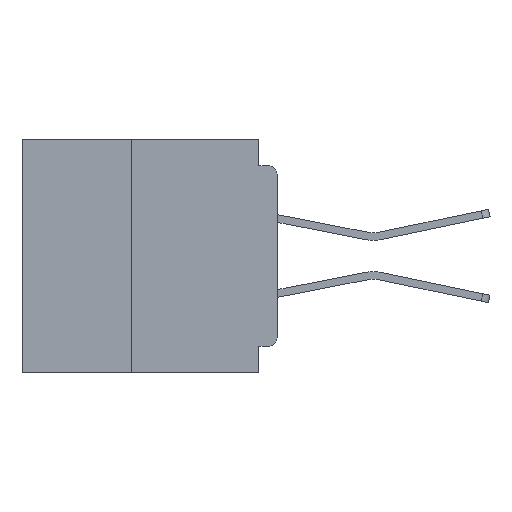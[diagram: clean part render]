
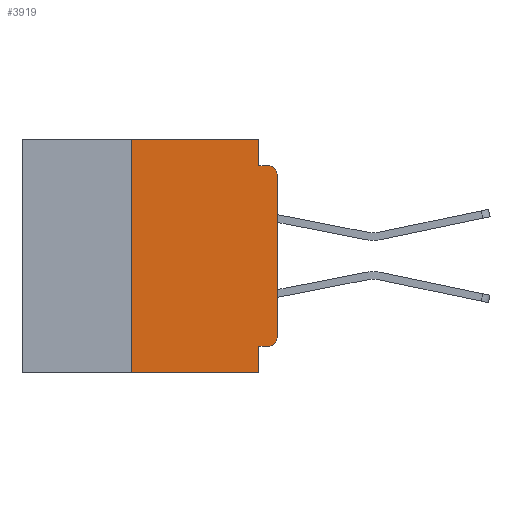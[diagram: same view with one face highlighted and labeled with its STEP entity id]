
A CAD part, left-side view. The second image highlights one B-rep face of the part: STEP entity #3919.
In plain terms, the highlighted planar face has unit normal (-1, 0, 0).
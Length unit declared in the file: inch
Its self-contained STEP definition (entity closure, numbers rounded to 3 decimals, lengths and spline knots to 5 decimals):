
#344 = DIRECTION ( 'NONE',  ( 0., 0., -1. ) ) ;
#1067 = CARTESIAN_POINT ( 'NONE',  ( 0., 0., -0.06 ) ) ;
#1111 = VECTOR ( 'NONE', #30399, 39.37008 ) ;
#1679 = VECTOR ( 'NONE', #43311, 39.37008 ) ;
#3634 = ORIENTED_EDGE ( 'NONE', *, *, #13479, .F. ) ;
#3635 = DIRECTION ( 'NONE',  ( 0., 0., 1. ) ) ;
#3919 = ADVANCED_FACE ( 'NONE', ( #28523 ), #49571, .F. ) ;
#3996 = VERTEX_POINT ( 'NONE', #1067 ) ;
#8938 = LINE ( 'NONE', #18709, #19869 ) ;
#9165 = ORIENTED_EDGE ( 'NONE', *, *, #11677, .T. ) ;
#9570 = VERTEX_POINT ( 'NONE', #10868 ) ;
#10157 = VERTEX_POINT ( 'NONE', #14753 ) ;
#10261 = VECTOR ( 'NONE', #28256, 39.37008 ) ;
#10330 = VERTEX_POINT ( 'NONE', #11657 ) ;
#10868 = CARTESIAN_POINT ( 'NONE',  ( 0., 0.031, -0.045 ) ) ;
#11498 = CARTESIAN_POINT ( 'NONE',  ( 0., 0.031, 0. ) ) ;
#11657 = CARTESIAN_POINT ( 'NONE',  ( 0., 0.25, -0.4 ) ) ;
#11677 = EDGE_CURVE ( 'NONE', #28107, #3996, #35769, .T. ) ;
#12485 = CARTESIAN_POINT ( 'NONE',  ( 0., 0., -0.355 ) ) ;
#13479 = EDGE_CURVE ( 'NONE', #10157, #34674, #44838, .T. ) ;
#14753 = CARTESIAN_POINT ( 'NONE',  ( 0., 0.031, -0.355 ) ) ;
#15132 = CIRCLE ( 'NONE', #24941, 0.015 ) ;
#15340 = VECTOR ( 'NONE', #19314, 39.37008 ) ;
#17883 = LINE ( 'NONE', #39965, #27533 ) ;
#17892 = CARTESIAN_POINT ( 'NONE',  ( 0., 0.031, -0.4 ) ) ;
#18213 = CARTESIAN_POINT ( 'NONE',  ( 0., 0.015, -0.06 ) ) ;
#18709 = CARTESIAN_POINT ( 'NONE',  ( 0., 0.437, -0.4 ) ) ;
#19314 = DIRECTION ( 'NONE',  ( 0., 0., -1. ) ) ;
#19401 = VERTEX_POINT ( 'NONE', #26778 ) ;
#19869 = VECTOR ( 'NONE', #51497, 39.37008 ) ;
#20520 = DIRECTION ( 'NONE',  ( -1., 0., 0. ) ) ;
#22367 = DIRECTION ( 'NONE',  ( 0., 0., -1. ) ) ;
#22572 = ORIENTED_EDGE ( 'NONE', *, *, #42829, .F. ) ;
#22783 = ORIENTED_EDGE ( 'NONE', *, *, #25058, .T. ) ;
#23039 = ORIENTED_EDGE ( 'NONE', *, *, #51275, .F. ) ;
#23736 = ORIENTED_EDGE ( 'NONE', *, *, #46332, .T. ) ;
#24015 = AXIS2_PLACEMENT_3D ( 'NONE', #45073, #20520, #49177 ) ;
#24412 = ORIENTED_EDGE ( 'NONE', *, *, #48598, .T. ) ;
#24941 = AXIS2_PLACEMENT_3D ( 'NONE', #18213, #46890, #22367 ) ;
#25039 = DIRECTION ( 'NONE',  ( 1., 0., 0. ) ) ;
#25058 = EDGE_CURVE ( 'NONE', #10330, #34674, #8938, .T. ) ;
#26287 = LINE ( 'NONE', #52094, #15340 ) ;
#26581 = AXIS2_PLACEMENT_3D ( 'NONE', #41367, #25039, #344 ) ;
#26778 = CARTESIAN_POINT ( 'NONE',  ( 0., 0.25, 0. ) ) ;
#27533 = VECTOR ( 'NONE', #44059, 39.37008 ) ;
#27597 = EDGE_LOOP ( 'NONE', ( #9165, #23736, #44191, #23039, #45460, #22572, #22783, #3634, #50685, #24412 ) ) ;
#27775 = VECTOR ( 'NONE', #3635, 39.37008 ) ;
#28107 = VERTEX_POINT ( 'NONE', #51499 ) ;
#28239 = VERTEX_POINT ( 'NONE', #11498 ) ;
#28250 = CARTESIAN_POINT ( 'NONE',  ( 0., 0.25, -0.4 ) ) ;
#28256 = DIRECTION ( 'NONE',  ( 0., -1., 0. ) ) ;
#28523 = FACE_OUTER_BOUND ( 'NONE', #27597, .T. ) ;
#29038 = LINE ( 'NONE', #28250, #27775 ) ;
#30320 = CARTESIAN_POINT ( 'NONE',  ( 0., 0.015, -0.045 ) ) ;
#30399 = DIRECTION ( 'NONE',  ( 0., 0., -1. ) ) ;
#30941 = CARTESIAN_POINT ( 'NONE',  ( 0., 0., 0. ) ) ;
#32846 = CIRCLE ( 'NONE', #24015, 0.015 ) ;
#33433 = VERTEX_POINT ( 'NONE', #44374 ) ;
#34674 = VERTEX_POINT ( 'NONE', #17892 ) ;
#34954 = EDGE_CURVE ( 'NONE', #19401, #28239, #17883, .T. ) ;
#35769 = LINE ( 'NONE', #30941, #1679 ) ;
#38579 = VECTOR ( 'NONE', #41229, 39.37008 ) ;
#39965 = CARTESIAN_POINT ( 'NONE',  ( 0., 0.437, 0. ) ) ;
#41229 = DIRECTION ( 'NONE',  ( 0., 1., 0. ) ) ;
#41367 = CARTESIAN_POINT ( 'NONE',  ( 0., 0.437, 0. ) ) ;
#42829 = EDGE_CURVE ( 'NONE', #10330, #19401, #29038, .T. ) ;
#43008 = LINE ( 'NONE', #52763, #10261 ) ;
#43311 = DIRECTION ( 'NONE',  ( 0., 0., 1. ) ) ;
#43675 = EDGE_CURVE ( 'NONE', #33433, #10157, #49434, .T. ) ;
#44059 = DIRECTION ( 'NONE',  ( 0., -1., 0. ) ) ;
#44191 = ORIENTED_EDGE ( 'NONE', *, *, #44253, .F. ) ;
#44253 = EDGE_CURVE ( 'NONE', #9570, #45217, #43008, .T. ) ;
#44374 = CARTESIAN_POINT ( 'NONE',  ( 0., 0.015, -0.355 ) ) ;
#44838 = LINE ( 'NONE', #50780, #1111 ) ;
#45073 = CARTESIAN_POINT ( 'NONE',  ( 0., 0.015, -0.34 ) ) ;
#45217 = VERTEX_POINT ( 'NONE', #30320 ) ;
#45460 = ORIENTED_EDGE ( 'NONE', *, *, #34954, .F. ) ;
#46332 = EDGE_CURVE ( 'NONE', #3996, #45217, #15132, .T. ) ;
#46890 = DIRECTION ( 'NONE',  ( -1., 0., 0. ) ) ;
#48598 = EDGE_CURVE ( 'NONE', #33433, #28107, #32846, .T. ) ;
#49177 = DIRECTION ( 'NONE',  ( 0., 0., -1. ) ) ;
#49434 = LINE ( 'NONE', #12485, #38579 ) ;
#49571 = PLANE ( 'NONE',  #26581 ) ;
#50685 = ORIENTED_EDGE ( 'NONE', *, *, #43675, .F. ) ;
#50780 = CARTESIAN_POINT ( 'NONE',  ( 0., 0.031, -0.4 ) ) ;
#51275 = EDGE_CURVE ( 'NONE', #28239, #9570, #26287, .T. ) ;
#51497 = DIRECTION ( 'NONE',  ( 0., -1., 0. ) ) ;
#51499 = CARTESIAN_POINT ( 'NONE',  ( 0., 0., -0.34 ) ) ;
#52094 = CARTESIAN_POINT ( 'NONE',  ( 0., 0.031, 0. ) ) ;
#52763 = CARTESIAN_POINT ( 'NONE',  ( 0., 0., -0.045 ) ) ;
